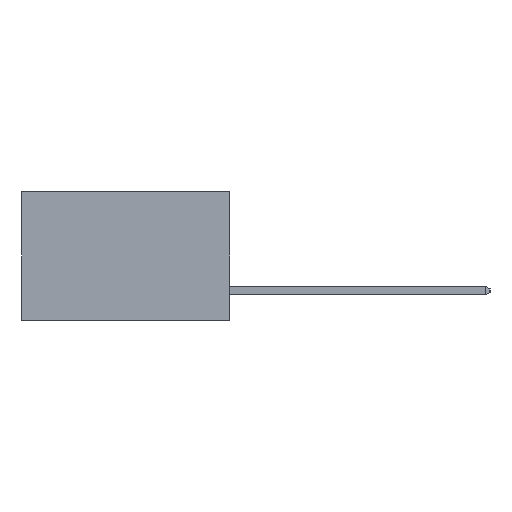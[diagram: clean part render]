
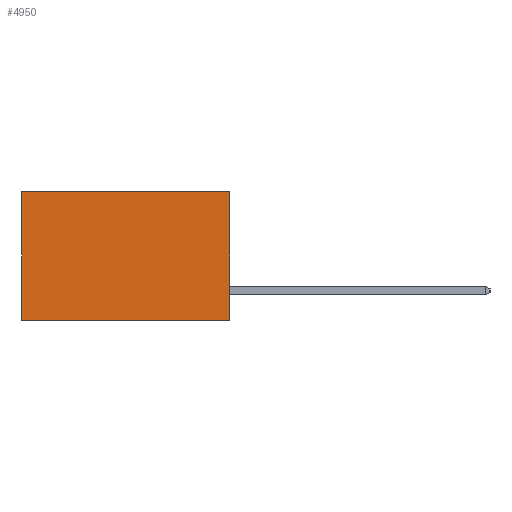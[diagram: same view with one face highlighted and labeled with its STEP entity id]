
A CAD part, left-side view. The second image highlights one B-rep face of the part: STEP entity #4950.
In plain terms, the highlighted planar face has unit normal (-1, 0, 0).
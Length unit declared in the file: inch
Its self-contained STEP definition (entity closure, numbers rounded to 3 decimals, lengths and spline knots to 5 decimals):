
#216 = EDGE_CURVE ( 'NONE', #10219, #7968, #2610, .T. ) ;
#897 = VERTEX_POINT ( 'NONE', #7202 ) ;
#1064 = DIRECTION ( 'NONE',  ( 0., 0., -1. ) ) ;
#1202 = LINE ( 'NONE', #9180, #3949 ) ;
#1399 = AXIS2_PLACEMENT_3D ( 'NONE', #10877, #9050, #2022 ) ;
#1637 = ORIENTED_EDGE ( 'NONE', *, *, #4000, .F. ) ;
#1648 = ORIENTED_EDGE ( 'NONE', *, *, #2210, .F. ) ;
#1738 = ORIENTED_EDGE ( 'NONE', *, *, #216, .T. ) ;
#2022 = DIRECTION ( 'NONE',  ( 0., 0., -1. ) ) ;
#2088 = FACE_OUTER_BOUND ( 'NONE', #2404, .T. ) ;
#2210 = EDGE_CURVE ( 'NONE', #10219, #6773, #3288, .T. ) ;
#2404 = EDGE_LOOP ( 'NONE', ( #10780, #1637, #1648, #1738 ) ) ;
#2610 = LINE ( 'NONE', #2769, #5045 ) ;
#2769 = CARTESIAN_POINT ( 'NONE',  ( 0.298, 0., 0. ) ) ;
#2894 = VECTOR ( 'NONE', #1064, 39.37008 ) ;
#3248 = CARTESIAN_POINT ( 'NONE',  ( 0.298, 0., 0. ) ) ;
#3274 = CARTESIAN_POINT ( 'NONE',  ( 0.298, 0., 0. ) ) ;
#3288 = LINE ( 'NONE', #3274, #9901 ) ;
#3706 = DIRECTION ( 'NONE',  ( 0., 0., -1. ) ) ;
#3949 = VECTOR ( 'NONE', #8225, 39.37008 ) ;
#4000 = EDGE_CURVE ( 'NONE', #6773, #897, #1202, .T. ) ;
#4629 = CARTESIAN_POINT ( 'NONE',  ( 0.298, 0., -0.37 ) ) ;
#4950 = ADVANCED_FACE ( 'NONE', ( #2088 ), #10620, .F. ) ;
#5045 = VECTOR ( 'NONE', #10930, 39.37008 ) ;
#5310 = LINE ( 'NONE', #9817, #2894 ) ;
#6773 = VERTEX_POINT ( 'NONE', #4629 ) ;
#7202 = CARTESIAN_POINT ( 'NONE',  ( 0.298, 0.6, -0.37 ) ) ;
#7968 = VERTEX_POINT ( 'NONE', #10658 ) ;
#8225 = DIRECTION ( 'NONE',  ( 0., 1., 0. ) ) ;
#9050 = DIRECTION ( 'NONE',  ( 1., 0., 0. ) ) ;
#9180 = CARTESIAN_POINT ( 'NONE',  ( 0.298, 0., -0.37 ) ) ;
#9817 = CARTESIAN_POINT ( 'NONE',  ( 0.298, 0.6, 0. ) ) ;
#9901 = VECTOR ( 'NONE', #3706, 39.37008 ) ;
#9917 = EDGE_CURVE ( 'NONE', #7968, #897, #5310, .T. ) ;
#10219 = VERTEX_POINT ( 'NONE', #3248 ) ;
#10620 = PLANE ( 'NONE',  #1399 ) ;
#10658 = CARTESIAN_POINT ( 'NONE',  ( 0.298, 0.6, 0. ) ) ;
#10780 = ORIENTED_EDGE ( 'NONE', *, *, #9917, .T. ) ;
#10877 = CARTESIAN_POINT ( 'NONE',  ( 0.298, 0., 0. ) ) ;
#10930 = DIRECTION ( 'NONE',  ( 0., 1., 0. ) ) ;
